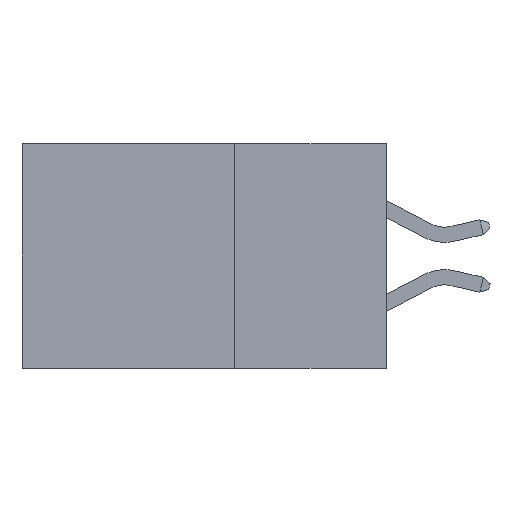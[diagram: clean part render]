
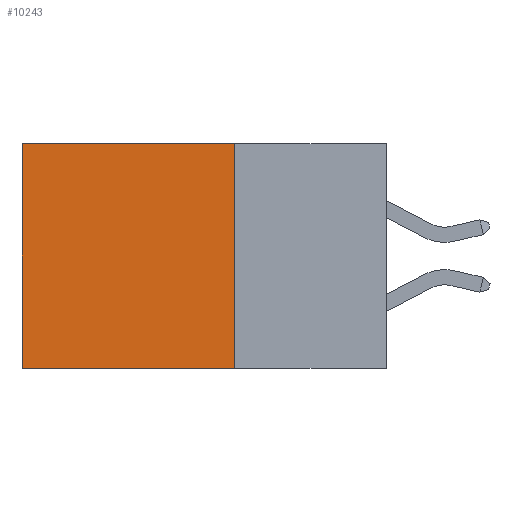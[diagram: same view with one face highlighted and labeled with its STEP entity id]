
A CAD part, left-side view. The second image highlights one B-rep face of the part: STEP entity #10243.
In plain terms, the highlighted planar face has unit normal (-1, 0, 0).
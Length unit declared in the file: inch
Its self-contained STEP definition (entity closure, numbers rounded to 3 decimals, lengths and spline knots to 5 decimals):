
#386 = ORIENTED_EDGE ( 'NONE', *, *, #3505, .T. ) ;
#464 = VERTEX_POINT ( 'NONE', #4838 ) ;
#952 = LINE ( 'NONE', #8092, #3271 ) ;
#1026 = LINE ( 'NONE', #9944, #9610 ) ;
#1055 = FACE_OUTER_BOUND ( 'NONE', #4048, .T. ) ;
#1056 = VERTEX_POINT ( 'NONE', #4168 ) ;
#2653 = PLANE ( 'NONE',  #6030 ) ;
#3271 = VECTOR ( 'NONE', #6989, 39.37008 ) ;
#3434 = ORIENTED_EDGE ( 'NONE', *, *, #7203, .F. ) ;
#3505 = EDGE_CURVE ( 'NONE', #4642, #464, #1026, .T. ) ;
#3564 = VECTOR ( 'NONE', #12197, 39.37008 ) ;
#3670 = DIRECTION ( 'NONE',  ( 1., 0., 0. ) ) ;
#3785 = DIRECTION ( 'NONE',  ( 0., 0., -1. ) ) ;
#3842 = VECTOR ( 'NONE', #9846, 39.37008 ) ;
#4048 = EDGE_LOOP ( 'NONE', ( #9848, #3434, #5069, #386 ) ) ;
#4097 = DIRECTION ( 'NONE',  ( 0., 1., 0. ) ) ;
#4168 = CARTESIAN_POINT ( 'NONE',  ( 0.298, 0.6, -0.37 ) ) ;
#4642 = VERTEX_POINT ( 'NONE', #10937 ) ;
#4800 = CARTESIAN_POINT ( 'NONE',  ( 0.298, 0.25, -0.37 ) ) ;
#4838 = CARTESIAN_POINT ( 'NONE',  ( 0.298, 0.6, 0. ) ) ;
#5069 = ORIENTED_EDGE ( 'NONE', *, *, #8573, .F. ) ;
#5165 = CARTESIAN_POINT ( 'NONE',  ( 0.298, 0.6, 0. ) ) ;
#5485 = VERTEX_POINT ( 'NONE', #4800 ) ;
#5662 = CARTESIAN_POINT ( 'NONE',  ( 0.298, 0.25, 0. ) ) ;
#5990 = LINE ( 'NONE', #7303, #3564 ) ;
#6030 = AXIS2_PLACEMENT_3D ( 'NONE', #5662, #3670, #3785 ) ;
#6989 = DIRECTION ( 'NONE',  ( 0., 1., 0. ) ) ;
#7203 = EDGE_CURVE ( 'NONE', #5485, #1056, #952, .T. ) ;
#7303 = CARTESIAN_POINT ( 'NONE',  ( 0.298, 0.25, 0. ) ) ;
#8092 = CARTESIAN_POINT ( 'NONE',  ( 0.298, 0.25, -0.37 ) ) ;
#8303 = LINE ( 'NONE', #5165, #3842 ) ;
#8573 = EDGE_CURVE ( 'NONE', #4642, #5485, #5990, .T. ) ;
#9496 = EDGE_CURVE ( 'NONE', #464, #1056, #8303, .T. ) ;
#9610 = VECTOR ( 'NONE', #4097, 39.37008 ) ;
#9846 = DIRECTION ( 'NONE',  ( 0., 0., -1. ) ) ;
#9848 = ORIENTED_EDGE ( 'NONE', *, *, #9496, .T. ) ;
#9944 = CARTESIAN_POINT ( 'NONE',  ( 0.298, 0.25, 0. ) ) ;
#10243 = ADVANCED_FACE ( 'NONE', ( #1055 ), #2653, .F. ) ;
#10937 = CARTESIAN_POINT ( 'NONE',  ( 0.298, 0.25, 0. ) ) ;
#12197 = DIRECTION ( 'NONE',  ( 0., 0., -1. ) ) ;
